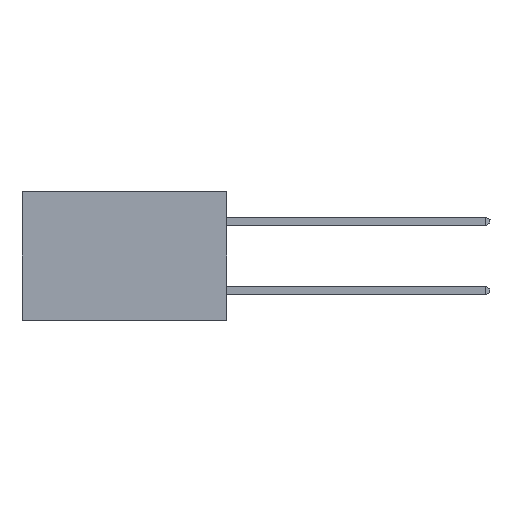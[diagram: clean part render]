
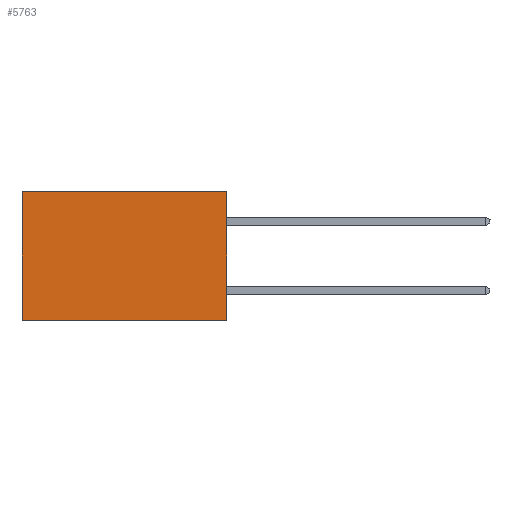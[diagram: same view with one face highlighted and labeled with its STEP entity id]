
A CAD part, left-side view. The second image highlights one B-rep face of the part: STEP entity #5763.
In plain terms, the highlighted planar face has unit normal (-1, 0, 0).
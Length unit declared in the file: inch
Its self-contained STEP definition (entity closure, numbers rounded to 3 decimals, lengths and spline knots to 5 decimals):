
#308 = ORIENTED_EDGE ( 'NONE', *, *, #5670, .F. ) ;
#620 = EDGE_CURVE ( 'NONE', #11513, #4730, #2658, .T. ) ;
#1054 = VERTEX_POINT ( 'NONE', #7743 ) ;
#1664 = ORIENTED_EDGE ( 'NONE', *, *, #7349, .T. ) ;
#2658 = LINE ( 'NONE', #12309, #7896 ) ;
#2764 = LINE ( 'NONE', #7132, #5906 ) ;
#3387 = CARTESIAN_POINT ( 'NONE',  ( 0.277, 0., -0.37 ) ) ;
#3537 = DIRECTION ( 'NONE',  ( 0., 0., -1. ) ) ;
#3555 = CARTESIAN_POINT ( 'NONE',  ( 0.277, 0.59, -0.37 ) ) ;
#3761 = LINE ( 'NONE', #11141, #5862 ) ;
#4730 = VERTEX_POINT ( 'NONE', #12145 ) ;
#4904 = EDGE_LOOP ( 'NONE', ( #9658, #8593, #308, #1664 ) ) ;
#5254 = VERTEX_POINT ( 'NONE', #9170 ) ;
#5670 = EDGE_CURVE ( 'NONE', #5254, #11513, #2764, .T. ) ;
#5763 = ADVANCED_FACE ( 'NONE', ( #11729 ), #6435, .F. ) ;
#5862 = VECTOR ( 'NONE', #11580, 39.37008 ) ;
#5906 = VECTOR ( 'NONE', #7134, 39.37008 ) ;
#6218 = EDGE_CURVE ( 'NONE', #1054, #4730, #9119, .T. ) ;
#6335 = AXIS2_PLACEMENT_3D ( 'NONE', #6440, #6391, #6379 ) ;
#6367 = VECTOR ( 'NONE', #3537, 39.37008 ) ;
#6379 = DIRECTION ( 'NONE',  ( 0., 0., -1. ) ) ;
#6391 = DIRECTION ( 'NONE',  ( 1., 0., 0. ) ) ;
#6435 = PLANE ( 'NONE',  #6335 ) ;
#6440 = CARTESIAN_POINT ( 'NONE',  ( 0.277, 0., -0.37 ) ) ;
#7132 = CARTESIAN_POINT ( 'NONE',  ( 0.277, 0., -0.37 ) ) ;
#7134 = DIRECTION ( 'NONE',  ( 0., 0., -1. ) ) ;
#7349 = EDGE_CURVE ( 'NONE', #5254, #1054, #3761, .T. ) ;
#7743 = CARTESIAN_POINT ( 'NONE',  ( 0.277, 0.59, 0. ) ) ;
#7896 = VECTOR ( 'NONE', #13218, 39.37008 ) ;
#8593 = ORIENTED_EDGE ( 'NONE', *, *, #620, .F. ) ;
#9119 = LINE ( 'NONE', #3555, #6367 ) ;
#9170 = CARTESIAN_POINT ( 'NONE',  ( 0.277, 0., 0. ) ) ;
#9658 = ORIENTED_EDGE ( 'NONE', *, *, #6218, .T. ) ;
#11141 = CARTESIAN_POINT ( 'NONE',  ( 0.277, 0., 0. ) ) ;
#11513 = VERTEX_POINT ( 'NONE', #3387 ) ;
#11580 = DIRECTION ( 'NONE',  ( 0., 1., 0. ) ) ;
#11729 = FACE_OUTER_BOUND ( 'NONE', #4904, .T. ) ;
#12145 = CARTESIAN_POINT ( 'NONE',  ( 0.277, 0.59, -0.37 ) ) ;
#12309 = CARTESIAN_POINT ( 'NONE',  ( 0.277, 0., -0.37 ) ) ;
#13218 = DIRECTION ( 'NONE',  ( 0., 1., 0. ) ) ;
